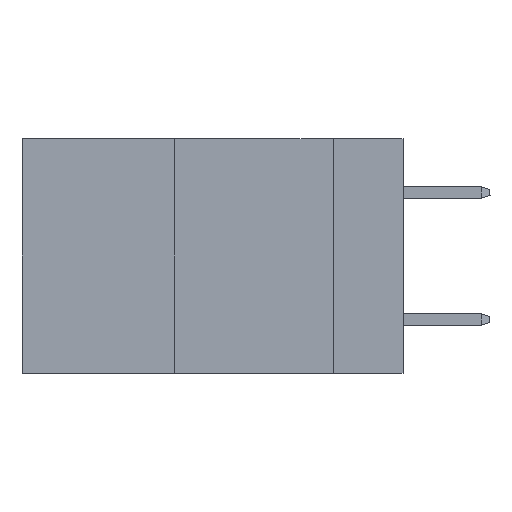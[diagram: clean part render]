
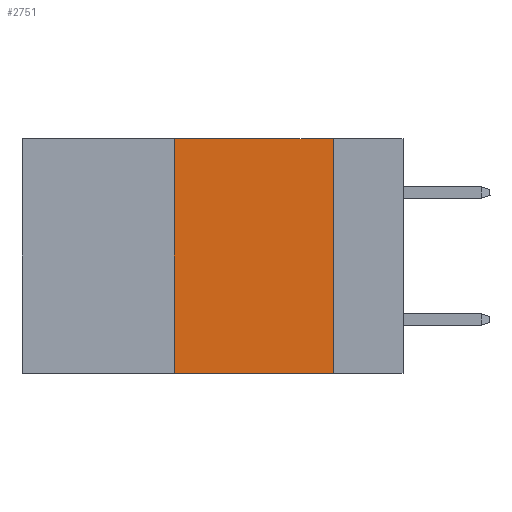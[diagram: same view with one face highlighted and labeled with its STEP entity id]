
A CAD part, left-side view. The second image highlights one B-rep face of the part: STEP entity #2751.
In plain terms, the highlighted planar face has unit normal (-1, 0, 0).
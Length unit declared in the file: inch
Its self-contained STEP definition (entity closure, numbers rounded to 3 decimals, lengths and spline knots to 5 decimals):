
#792 = VERTEX_POINT ( 'NONE', #4085 ) ;
#1043 = ORIENTED_EDGE ( 'NONE', *, *, #8234, .F. ) ;
#1237 = CARTESIAN_POINT ( 'NONE',  ( 0., 0.36, 0. ) ) ;
#1368 = LINE ( 'NONE', #5389, #7156 ) ;
#1504 = VERTEX_POINT ( 'NONE', #2537 ) ;
#1761 = EDGE_CURVE ( 'NONE', #1504, #792, #10232, .T. ) ;
#1888 = CARTESIAN_POINT ( 'NONE',  ( 0., 0.36, 0. ) ) ;
#2164 = CARTESIAN_POINT ( 'NONE',  ( 0., 0.6, -0.37 ) ) ;
#2537 = CARTESIAN_POINT ( 'NONE',  ( 0., 0.36, -0.37 ) ) ;
#2578 = DIRECTION ( 'NONE',  ( 0., 0., 1. ) ) ;
#2751 = ADVANCED_FACE ( 'NONE', ( #6299 ), #9532, .F. ) ;
#3046 = DIRECTION ( 'NONE',  ( 0., -1., 0. ) ) ;
#3354 = EDGE_CURVE ( 'NONE', #1504, #7398, #9083, .T. ) ;
#3678 = DIRECTION ( 'NONE',  ( 0., -1., 0. ) ) ;
#3706 = ORIENTED_EDGE ( 'NONE', *, *, #3834, .F. ) ;
#3834 = EDGE_CURVE ( 'NONE', #9022, #792, #1368, .T. ) ;
#3877 = ORIENTED_EDGE ( 'NONE', *, *, #3354, .F. ) ;
#4085 = CARTESIAN_POINT ( 'NONE',  ( 0., 0.11, -0.37 ) ) ;
#4656 = DIRECTION ( 'NONE',  ( 0., 0., -1. ) ) ;
#4865 = VECTOR ( 'NONE', #2578, 39.37008 ) ;
#5231 = LINE ( 'NONE', #5372, #7248 ) ;
#5372 = CARTESIAN_POINT ( 'NONE',  ( 0., 0.6, 0. ) ) ;
#5389 = CARTESIAN_POINT ( 'NONE',  ( 0., 0.11, 0. ) ) ;
#6299 = FACE_OUTER_BOUND ( 'NONE', #7804, .T. ) ;
#6984 = DIRECTION ( 'NONE',  ( 1., 0., 0. ) ) ;
#7156 = VECTOR ( 'NONE', #8633, 39.37008 ) ;
#7248 = VECTOR ( 'NONE', #3046, 39.37008 ) ;
#7398 = VERTEX_POINT ( 'NONE', #1888 ) ;
#7804 = EDGE_LOOP ( 'NONE', ( #3706, #1043, #3877, #9995 ) ) ;
#8234 = EDGE_CURVE ( 'NONE', #7398, #9022, #5231, .T. ) ;
#8633 = DIRECTION ( 'NONE',  ( 0., 0., -1. ) ) ;
#8682 = CARTESIAN_POINT ( 'NONE',  ( 0., 0.6, 0. ) ) ;
#8892 = VECTOR ( 'NONE', #3678, 39.37008 ) ;
#9022 = VERTEX_POINT ( 'NONE', #9865 ) ;
#9083 = LINE ( 'NONE', #1237, #4865 ) ;
#9399 = AXIS2_PLACEMENT_3D ( 'NONE', #8682, #6984, #4656 ) ;
#9532 = PLANE ( 'NONE',  #9399 ) ;
#9865 = CARTESIAN_POINT ( 'NONE',  ( 0., 0.11, 0. ) ) ;
#9995 = ORIENTED_EDGE ( 'NONE', *, *, #1761, .T. ) ;
#10232 = LINE ( 'NONE', #2164, #8892 ) ;
